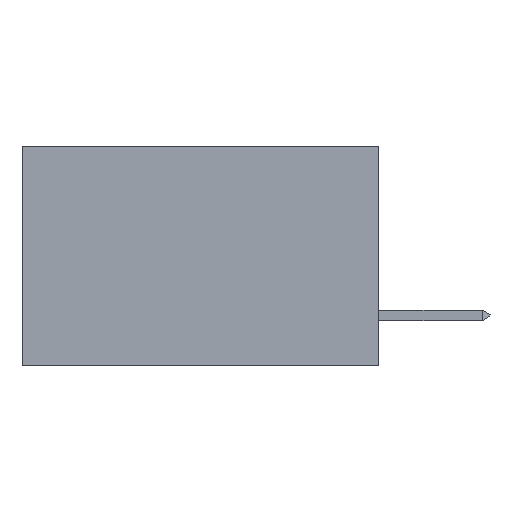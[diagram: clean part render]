
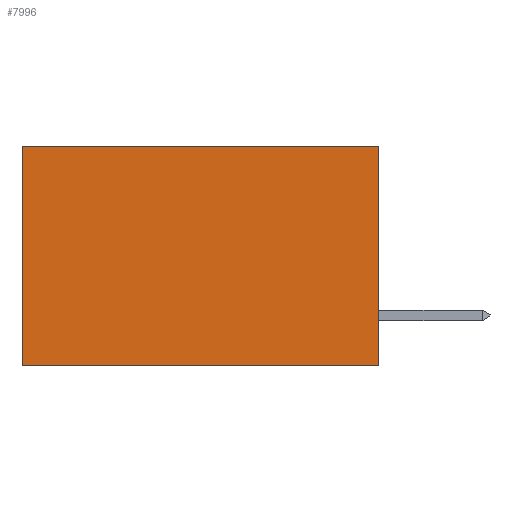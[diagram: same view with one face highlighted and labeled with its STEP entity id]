
A CAD part, left-side view. The second image highlights one B-rep face of the part: STEP entity #7996.
In plain terms, the highlighted planar face has unit normal (-1, 0, 0).
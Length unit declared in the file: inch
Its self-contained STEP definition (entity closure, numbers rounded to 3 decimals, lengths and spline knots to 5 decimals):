
#5 = ORIENTED_EDGE ( 'NONE', *, *, #9549, .F. ) ;
#395 = DIRECTION ( 'NONE',  ( 0., 0., -1. ) ) ;
#586 = DIRECTION ( 'NONE',  ( 1., 0., 0. ) ) ;
#772 = ORIENTED_EDGE ( 'NONE', *, *, #7252, .F. ) ;
#884 = LINE ( 'NONE', #5719, #6040 ) ;
#1699 = VERTEX_POINT ( 'NONE', #6084 ) ;
#2266 = LINE ( 'NONE', #3179, #5512 ) ;
#2618 = AXIS2_PLACEMENT_3D ( 'NONE', #3402, #586, #395 ) ;
#2828 = EDGE_CURVE ( 'NONE', #10403, #1699, #2266, .T. ) ;
#2962 = DIRECTION ( 'NONE',  ( 0., 0., -1. ) ) ;
#3179 = CARTESIAN_POINT ( 'NONE',  ( 0.2615, 0., 0. ) ) ;
#3402 = CARTESIAN_POINT ( 'NONE',  ( 0.2615, 0., -0.37 ) ) ;
#3470 = CARTESIAN_POINT ( 'NONE',  ( 0.2615, 0., -0.37 ) ) ;
#3832 = CARTESIAN_POINT ( 'NONE',  ( 0.2615, 0., -0.37 ) ) ;
#4320 = FACE_OUTER_BOUND ( 'NONE', #10699, .T. ) ;
#4807 = VECTOR ( 'NONE', #11304, 39.37008 ) ;
#4863 = DIRECTION ( 'NONE',  ( 0., 0., -1. ) ) ;
#5512 = VECTOR ( 'NONE', #10172, 39.37008 ) ;
#5719 = CARTESIAN_POINT ( 'NONE',  ( 0.2615, 0.6, -0.37 ) ) ;
#5857 = ORIENTED_EDGE ( 'NONE', *, *, #11486, .T. ) ;
#6040 = VECTOR ( 'NONE', #4863, 39.37008 ) ;
#6084 = CARTESIAN_POINT ( 'NONE',  ( 0.2615, 0.6, 0. ) ) ;
#7112 = CARTESIAN_POINT ( 'NONE',  ( 0.2615, 0., -0.37 ) ) ;
#7252 = EDGE_CURVE ( 'NONE', #10403, #12930, #9897, .T. ) ;
#7987 = VECTOR ( 'NONE', #2962, 39.37008 ) ;
#7996 = ADVANCED_FACE ( 'NONE', ( #4320 ), #9483, .F. ) ;
#8289 = LINE ( 'NONE', #3470, #4807 ) ;
#9483 = PLANE ( 'NONE',  #2618 ) ;
#9549 = EDGE_CURVE ( 'NONE', #12930, #11314, #8289, .T. ) ;
#9897 = LINE ( 'NONE', #3832, #7987 ) ;
#9906 = ORIENTED_EDGE ( 'NONE', *, *, #2828, .T. ) ;
#10141 = CARTESIAN_POINT ( 'NONE',  ( 0.2615, 0., 0. ) ) ;
#10172 = DIRECTION ( 'NONE',  ( 0., 1., 0. ) ) ;
#10403 = VERTEX_POINT ( 'NONE', #10141 ) ;
#10549 = CARTESIAN_POINT ( 'NONE',  ( 0.2615, 0.6, -0.37 ) ) ;
#10699 = EDGE_LOOP ( 'NONE', ( #5857, #5, #772, #9906 ) ) ;
#11304 = DIRECTION ( 'NONE',  ( 0., 1., 0. ) ) ;
#11314 = VERTEX_POINT ( 'NONE', #10549 ) ;
#11486 = EDGE_CURVE ( 'NONE', #1699, #11314, #884, .T. ) ;
#12930 = VERTEX_POINT ( 'NONE', #7112 ) ;
